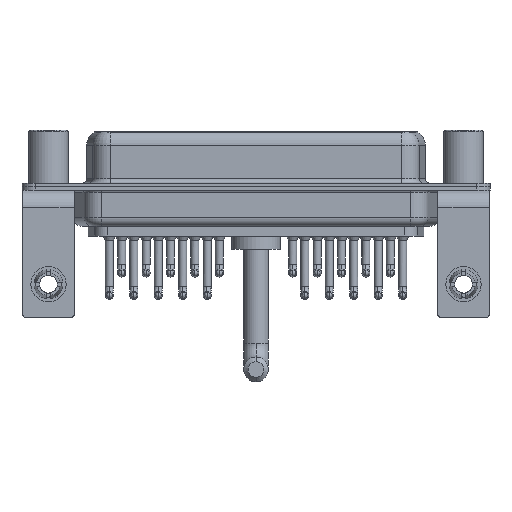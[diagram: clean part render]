
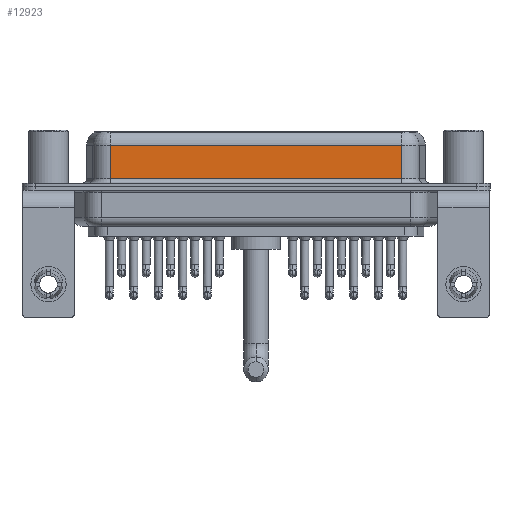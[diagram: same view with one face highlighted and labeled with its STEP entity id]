
A CAD part, front view. The second image highlights one B-rep face of the part: STEP entity #12923.
In plain terms, the highlighted planar face has unit normal (0, -1, 0).
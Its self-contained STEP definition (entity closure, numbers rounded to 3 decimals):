
#556 = ORIENTED_EDGE ( 'NONE', *, *, #20030, .T. ) ;
#3670 = DIRECTION ( 'NONE',  ( 1., 0., 0. ) ) ;
#5136 = AXIS2_PLACEMENT_3D ( 'NONE', #8177, #22182, #24301 ) ;
#5297 = LINE ( 'NONE', #21037, #20957 ) ;
#6966 = VERTEX_POINT ( 'NONE', #24865 ) ;
#7202 = ORIENTED_EDGE ( 'NONE', *, *, #18725, .T. ) ;
#8177 = CARTESIAN_POINT ( 'NONE',  ( 40.037, -3.95, 6.4 ) ) ;
#8231 = LINE ( 'NONE', #24085, #18889 ) ;
#8741 = LINE ( 'NONE', #16811, #13257 ) ;
#10662 = LINE ( 'NONE', #25774, #22147 ) ;
#11923 = ORIENTED_EDGE ( 'NONE', *, *, #24465, .F. ) ;
#12704 = ORIENTED_EDGE ( 'NONE', *, *, #23217, .T. ) ;
#12923 = ADVANCED_FACE ( 'NONE', ( #16243 ), #20195, .F. ) ;
#12963 = VERTEX_POINT ( 'NONE', #26026 ) ;
#13174 = VERTEX_POINT ( 'NONE', #15077 ) ;
#13257 = VECTOR ( 'NONE', #24882, 1000. ) ;
#15077 = CARTESIAN_POINT ( 'NONE',  ( 40.037, -3.95, 0.9 ) ) ;
#15670 = CARTESIAN_POINT ( 'NONE',  ( 7.013, -3.95, 4.65 ) ) ;
#16243 = FACE_OUTER_BOUND ( 'NONE', #20339, .T. ) ;
#16294 = DIRECTION ( 'NONE',  ( 0., 0., -1. ) ) ;
#16811 = CARTESIAN_POINT ( 'NONE',  ( 40.037, -3.95, 4.65 ) ) ;
#16947 = VERTEX_POINT ( 'NONE', #15670 ) ;
#17075 = DIRECTION ( 'NONE',  ( 0., 0., -1. ) ) ;
#18725 = EDGE_CURVE ( 'NONE', #6966, #16947, #8741, .T. ) ;
#18889 = VECTOR ( 'NONE', #16294, 1000. ) ;
#20030 = EDGE_CURVE ( 'NONE', #12963, #13174, #10662, .T. ) ;
#20195 = PLANE ( 'NONE',  #5136 ) ;
#20339 = EDGE_LOOP ( 'NONE', ( #11923, #7202, #12704, #556 ) ) ;
#20957 = VECTOR ( 'NONE', #17075, 1000. ) ;
#21037 = CARTESIAN_POINT ( 'NONE',  ( 7.013, -3.95, 6.4 ) ) ;
#22147 = VECTOR ( 'NONE', #3670, 1000. ) ;
#22182 = DIRECTION ( 'NONE',  ( 0., 1., 0. ) ) ;
#23217 = EDGE_CURVE ( 'NONE', #16947, #12963, #5297, .T. ) ;
#24085 = CARTESIAN_POINT ( 'NONE',  ( 40.037, -3.95, 6.4 ) ) ;
#24301 = DIRECTION ( 'NONE',  ( 0., 0., 1. ) ) ;
#24465 = EDGE_CURVE ( 'NONE', #6966, #13174, #8231, .T. ) ;
#24865 = CARTESIAN_POINT ( 'NONE',  ( 40.037, -3.95, 4.65 ) ) ;
#24882 = DIRECTION ( 'NONE',  ( -1., 0., 0. ) ) ;
#25774 = CARTESIAN_POINT ( 'NONE',  ( 40.037, -3.95, 0.9 ) ) ;
#26026 = CARTESIAN_POINT ( 'NONE',  ( 7.013, -3.95, 0.9 ) ) ;
